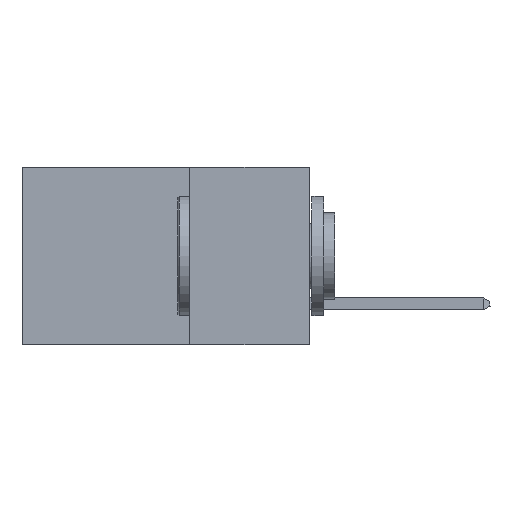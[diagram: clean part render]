
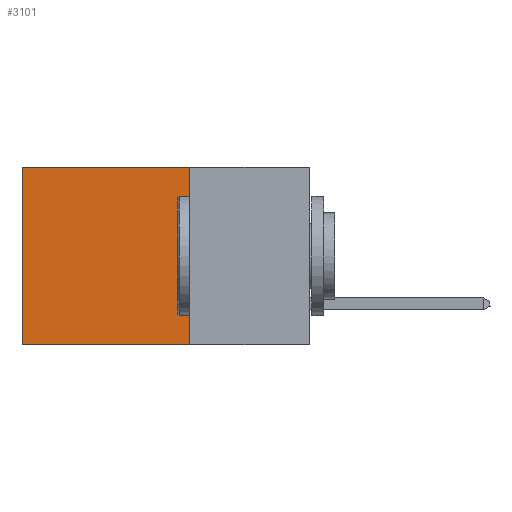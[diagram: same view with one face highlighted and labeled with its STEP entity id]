
A CAD part, left-side view. The second image highlights one B-rep face of the part: STEP entity #3101.
In plain terms, the highlighted planar face has unit normal (-1, 0, 0).
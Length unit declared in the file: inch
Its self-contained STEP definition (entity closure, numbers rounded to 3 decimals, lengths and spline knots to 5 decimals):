
#1791 = VECTOR ( 'NONE', #3340, 39.37008 ) ;
#3101 = ADVANCED_FACE ( 'NONE', ( #13465 ), #12139, .F. ) ;
#3340 = DIRECTION ( 'NONE',  ( 0., 0., -1. ) ) ;
#4126 = DIRECTION ( 'NONE',  ( 0., 1., 0. ) ) ;
#4267 = VECTOR ( 'NONE', #13668, 39.37008 ) ;
#4848 = LINE ( 'NONE', #22648, #4267 ) ;
#5631 = EDGE_LOOP ( 'NONE', ( #17816, #14247, #17067, #15403 ) ) ;
#5707 = EDGE_CURVE ( 'NONE', #6678, #17784, #15107, .T. ) ;
#6678 = VERTEX_POINT ( 'NONE', #15549 ) ;
#7020 = VERTEX_POINT ( 'NONE', #12848 ) ;
#7046 = AXIS2_PLACEMENT_3D ( 'NONE', #11591, #11588, #11547 ) ;
#9688 = CARTESIAN_POINT ( 'NONE',  ( 0.2875, 0.25, 0. ) ) ;
#10514 = CARTESIAN_POINT ( 'NONE',  ( 0.2875, 0.6, 0. ) ) ;
#11307 = EDGE_CURVE ( 'NONE', #6678, #15786, #20404, .T. ) ;
#11547 = DIRECTION ( 'NONE',  ( 0., 0., -1. ) ) ;
#11583 = LINE ( 'NONE', #23311, #1791 ) ;
#11588 = DIRECTION ( 'NONE',  ( 1., 0., 0. ) ) ;
#11591 = CARTESIAN_POINT ( 'NONE',  ( 0.2875, 0.25, 0. ) ) ;
#12139 = PLANE ( 'NONE',  #7046 ) ;
#12304 = EDGE_CURVE ( 'NONE', #15786, #7020, #11583, .T. ) ;
#12749 = DIRECTION ( 'NONE',  ( 0., 0., -1. ) ) ;
#12848 = CARTESIAN_POINT ( 'NONE',  ( 0.2875, 0.6, -0.37 ) ) ;
#13465 = FACE_OUTER_BOUND ( 'NONE', #5631, .T. ) ;
#13668 = DIRECTION ( 'NONE',  ( 0., 1., 0. ) ) ;
#14247 = ORIENTED_EDGE ( 'NONE', *, *, #23370, .F. ) ;
#15107 = LINE ( 'NONE', #20092, #19340 ) ;
#15403 = ORIENTED_EDGE ( 'NONE', *, *, #11307, .T. ) ;
#15549 = CARTESIAN_POINT ( 'NONE',  ( 0.2875, 0.25, 0. ) ) ;
#15786 = VERTEX_POINT ( 'NONE', #10514 ) ;
#17067 = ORIENTED_EDGE ( 'NONE', *, *, #5707, .F. ) ;
#17473 = CARTESIAN_POINT ( 'NONE',  ( 0.2875, 0.25, -0.37 ) ) ;
#17784 = VERTEX_POINT ( 'NONE', #17473 ) ;
#17816 = ORIENTED_EDGE ( 'NONE', *, *, #12304, .T. ) ;
#19340 = VECTOR ( 'NONE', #12749, 39.37008 ) ;
#20092 = CARTESIAN_POINT ( 'NONE',  ( 0.2875, 0.25, 0. ) ) ;
#20404 = LINE ( 'NONE', #9688, #20956 ) ;
#20956 = VECTOR ( 'NONE', #4126, 39.37008 ) ;
#22648 = CARTESIAN_POINT ( 'NONE',  ( 0.2875, 0.25, -0.37 ) ) ;
#23311 = CARTESIAN_POINT ( 'NONE',  ( 0.2875, 0.6, 0. ) ) ;
#23370 = EDGE_CURVE ( 'NONE', #17784, #7020, #4848, .T. ) ;
